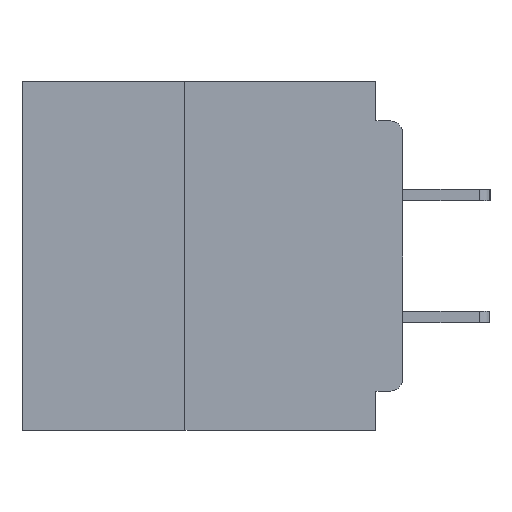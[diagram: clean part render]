
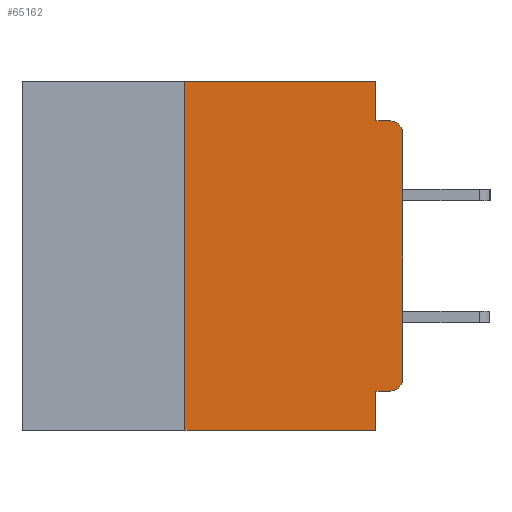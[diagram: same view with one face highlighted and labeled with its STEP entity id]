
A CAD part, left-side view. The second image highlights one B-rep face of the part: STEP entity #65162.
In plain terms, the highlighted planar face has unit normal (-1, 0, 0).
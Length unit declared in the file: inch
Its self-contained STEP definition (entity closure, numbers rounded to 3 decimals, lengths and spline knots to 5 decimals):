
#1233 = VERTEX_POINT ( 'NONE', #17671 ) ;
#1351 = CARTESIAN_POINT ( 'NONE',  ( 0., 0.015, -0.045 ) ) ;
#1480 = EDGE_CURVE ( 'NONE', #37099, #27671, #3142, .T. ) ;
#1842 = VECTOR ( 'NONE', #27854, 39.37008 ) ;
#2109 = DIRECTION ( 'NONE',  ( -1., 0., 0. ) ) ;
#3024 = EDGE_CURVE ( 'NONE', #22221, #5847, #58102, .T. ) ;
#3142 = LINE ( 'NONE', #10143, #4837 ) ;
#3533 = LINE ( 'NONE', #38466, #1842 ) ;
#4345 = VECTOR ( 'NONE', #60894, 39.37008 ) ;
#4532 = CARTESIAN_POINT ( 'NONE',  ( 0., 0.437, -0.4 ) ) ;
#4837 = VECTOR ( 'NONE', #15375, 39.37008 ) ;
#5847 = VERTEX_POINT ( 'NONE', #56400 ) ;
#9208 = DIRECTION ( 'NONE',  ( 0., -1., 0. ) ) ;
#9884 = DIRECTION ( 'NONE',  ( 0., -1., 0. ) ) ;
#10143 = CARTESIAN_POINT ( 'NONE',  ( 0., 0., 0. ) ) ;
#10279 = EDGE_CURVE ( 'NONE', #17607, #40439, #3533, .T. ) ;
#10469 = EDGE_CURVE ( 'NONE', #54205, #1233, #46444, .T. ) ;
#11664 = DIRECTION ( 'NONE',  ( -1., 0., 0. ) ) ;
#13507 = CARTESIAN_POINT ( 'NONE',  ( 0., 0.437, 0. ) ) ;
#13634 = ORIENTED_EDGE ( 'NONE', *, *, #64653, .F. ) ;
#14118 = FACE_OUTER_BOUND ( 'NONE', #38199, .T. ) ;
#14169 = EDGE_CURVE ( 'NONE', #54205, #5847, #32080, .T. ) ;
#15375 = DIRECTION ( 'NONE',  ( 0., 0., 1. ) ) ;
#15418 = ORIENTED_EDGE ( 'NONE', *, *, #14169, .T. ) ;
#16038 = VECTOR ( 'NONE', #48411, 39.37008 ) ;
#16329 = CARTESIAN_POINT ( 'NONE',  ( 0., 0.031, -0.4 ) ) ;
#16971 = EDGE_CURVE ( 'NONE', #62487, #22221, #17693, .T. ) ;
#17607 = VERTEX_POINT ( 'NONE', #42842 ) ;
#17671 = CARTESIAN_POINT ( 'NONE',  ( 0., 0.25, 0. ) ) ;
#17693 = LINE ( 'NONE', #32530, #16038 ) ;
#18736 = DIRECTION ( 'NONE',  ( 1., 0., 0. ) ) ;
#19516 = AXIS2_PLACEMENT_3D ( 'NONE', #43254, #11664, #48511 ) ;
#19839 = LINE ( 'NONE', #20848, #58500 ) ;
#20715 = LINE ( 'NONE', #40771, #34834 ) ;
#20848 = CARTESIAN_POINT ( 'NONE',  ( 0., 0.437, 0. ) ) ;
#21671 = CARTESIAN_POINT ( 'NONE',  ( 0., 0.015, -0.355 ) ) ;
#22221 = VERTEX_POINT ( 'NONE', #65558 ) ;
#24533 = ORIENTED_EDGE ( 'NONE', *, *, #61705, .F. ) ;
#24561 = ORIENTED_EDGE ( 'NONE', *, *, #66234, .T. ) ;
#26185 = DIRECTION ( 'NONE',  ( 0., -1., 0. ) ) ;
#27671 = VERTEX_POINT ( 'NONE', #37485 ) ;
#27854 = DIRECTION ( 'NONE',  ( 0., 0., -1. ) ) ;
#32080 = LINE ( 'NONE', #4532, #58319 ) ;
#32303 = DIRECTION ( 'NONE',  ( 0., 0., -1. ) ) ;
#32530 = CARTESIAN_POINT ( 'NONE',  ( 0., 0., -0.355 ) ) ;
#33792 = CARTESIAN_POINT ( 'NONE',  ( 0., 0.015, -0.34 ) ) ;
#34834 = VECTOR ( 'NONE', #9208, 39.37008 ) ;
#37099 = VERTEX_POINT ( 'NONE', #47207 ) ;
#37485 = CARTESIAN_POINT ( 'NONE',  ( 0., 0., -0.06 ) ) ;
#38199 = EDGE_LOOP ( 'NONE', ( #47205, #51507, #13634, #44160, #24533, #43122, #15418, #65096, #38784, #24561 ) ) ;
#38466 = CARTESIAN_POINT ( 'NONE',  ( 0., 0.031, 0. ) ) ;
#38784 = ORIENTED_EDGE ( 'NONE', *, *, #16971, .F. ) ;
#39085 = DIRECTION ( 'NONE',  ( 0., 0., -1. ) ) ;
#40439 = VERTEX_POINT ( 'NONE', #54106 ) ;
#40771 = CARTESIAN_POINT ( 'NONE',  ( 0., 0., -0.045 ) ) ;
#42582 = VECTOR ( 'NONE', #32303, 39.37008 ) ;
#42842 = CARTESIAN_POINT ( 'NONE',  ( 0., 0.031, 0. ) ) ;
#43122 = ORIENTED_EDGE ( 'NONE', *, *, #10469, .F. ) ;
#43254 = CARTESIAN_POINT ( 'NONE',  ( 0., 0.015, -0.06 ) ) ;
#44160 = ORIENTED_EDGE ( 'NONE', *, *, #10279, .F. ) ;
#45100 = PLANE ( 'NONE',  #52742 ) ;
#46444 = LINE ( 'NONE', #50420, #4345 ) ;
#47205 = ORIENTED_EDGE ( 'NONE', *, *, #1480, .T. ) ;
#47207 = CARTESIAN_POINT ( 'NONE',  ( 0., 0., -0.34 ) ) ;
#48411 = DIRECTION ( 'NONE',  ( 0., 1., 0. ) ) ;
#48511 = DIRECTION ( 'NONE',  ( 0., 0., -1. ) ) ;
#49388 = EDGE_CURVE ( 'NONE', #27671, #62572, #54123, .T. ) ;
#49884 = CARTESIAN_POINT ( 'NONE',  ( 0., 0.25, -0.4 ) ) ;
#50420 = CARTESIAN_POINT ( 'NONE',  ( 0., 0.25, -0.4 ) ) ;
#51055 = AXIS2_PLACEMENT_3D ( 'NONE', #33792, #2109, #39085 ) ;
#51507 = ORIENTED_EDGE ( 'NONE', *, *, #49388, .T. ) ;
#52742 = AXIS2_PLACEMENT_3D ( 'NONE', #13507, #18736, #55557 ) ;
#54106 = CARTESIAN_POINT ( 'NONE',  ( 0., 0.031, -0.045 ) ) ;
#54123 = CIRCLE ( 'NONE', #19516, 0.015 ) ;
#54205 = VERTEX_POINT ( 'NONE', #49884 ) ;
#54966 = CIRCLE ( 'NONE', #51055, 0.015 ) ;
#55557 = DIRECTION ( 'NONE',  ( 0., 0., -1. ) ) ;
#56400 = CARTESIAN_POINT ( 'NONE',  ( 0., 0.031, -0.4 ) ) ;
#58102 = LINE ( 'NONE', #16329, #42582 ) ;
#58319 = VECTOR ( 'NONE', #9884, 39.37008 ) ;
#58500 = VECTOR ( 'NONE', #26185, 39.37008 ) ;
#60894 = DIRECTION ( 'NONE',  ( 0., 0., 1. ) ) ;
#61705 = EDGE_CURVE ( 'NONE', #1233, #17607, #19839, .T. ) ;
#62487 = VERTEX_POINT ( 'NONE', #21671 ) ;
#62572 = VERTEX_POINT ( 'NONE', #1351 ) ;
#64653 = EDGE_CURVE ( 'NONE', #40439, #62572, #20715, .T. ) ;
#65096 = ORIENTED_EDGE ( 'NONE', *, *, #3024, .F. ) ;
#65162 = ADVANCED_FACE ( 'NONE', ( #14118 ), #45100, .F. ) ;
#65558 = CARTESIAN_POINT ( 'NONE',  ( 0., 0.031, -0.355 ) ) ;
#66234 = EDGE_CURVE ( 'NONE', #62487, #37099, #54966, .T. ) ;
